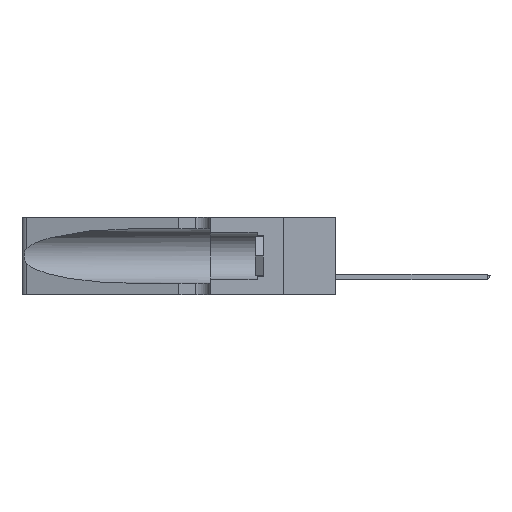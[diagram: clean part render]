
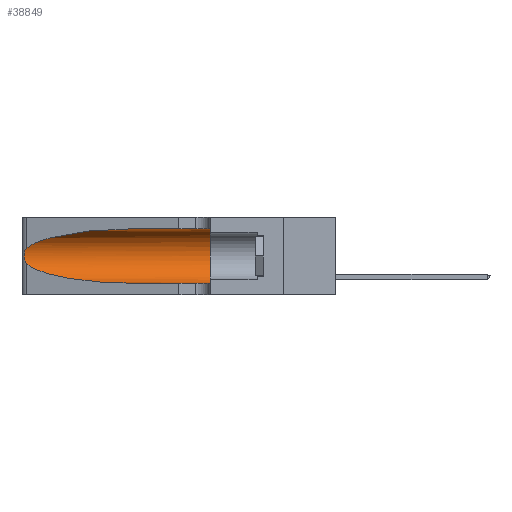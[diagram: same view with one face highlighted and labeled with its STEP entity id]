
A CAD part, left-side view. The second image highlights one B-rep face of the part: STEP entity #38849.
In plain terms, the highlighted cylindrical face has radius 3.308 mm (diameter 6.617 mm), a partial arc.
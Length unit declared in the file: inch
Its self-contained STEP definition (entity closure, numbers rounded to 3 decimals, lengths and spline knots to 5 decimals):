
#271 = DIRECTION ( 'NONE',  ( 0., 0., 1. ) ) ;
#306 = CARTESIAN_POINT ( 'NONE',  ( 0.1305, 0.72297, 0.05475 ) ) ;
#1023 = ORIENTED_EDGE ( 'NONE', *, *, #15821, .T. ) ;
#2103 =( BOUNDED_CURVE ( )  B_SPLINE_CURVE ( 3, ( #7111, #40244, #3651, #47270 ),
 .UNSPECIFIED., .F., .F. ) 
 B_SPLINE_CURVE_WITH_KNOTS ( ( 4, 4 ),
 ( 1.5708, 2.84003 ),
 .UNSPECIFIED. ) 
 CURVE ( )  GEOMETRIC_REPRESENTATION_ITEM ( )  RATIONAL_B_SPLINE_CURVE ( ( 1., 0.87, 0.87, 1. ) ) 
 REPRESENTATION_ITEM ( '' )  );
#2857 = CARTESIAN_POINT ( 'NONE',  ( 0.25487, 1.22718, 0.22369 ) ) ;
#3523 = CARTESIAN_POINT ( 'NONE',  ( 0.2373, 1.15595, 0.08982 ) ) ;
#3651 = CARTESIAN_POINT ( 'NONE',  ( 0.2373, 1.15595, 0.28018 ) ) ;
#4502 = ORIENTED_EDGE ( 'NONE', *, *, #24927, .T. ) ;
#5030 = B_SPLINE_CURVE_WITH_KNOTS ( 'NONE', 3,
 ( #2857, #31907, #13513, #46481, #17056, #17501, #28381, #6329, #13675, #28071, #20868, #9693, #6485, #28227 ),
 .UNSPECIFIED., .F., .F.,
 ( 4, 2, 2, 2, 2, 2, 4 ),
 ( 0., 0.00027, 0.00053, 0.00107, 0.0016, 0.00187, 0.00214 ),
 .UNSPECIFIED. ) ;
#6329 = CARTESIAN_POINT ( 'NONE',  ( 0.26075, 1.23896, 0.178 ) ) ;
#6485 = CARTESIAN_POINT ( 'NONE',  ( 0.25555, 1.22993, 0.14849 ) ) ;
#6826 = VERTEX_POINT ( 'NONE', #16613 ) ;
#7041 = ORIENTED_EDGE ( 'NONE', *, *, #30138, .T. ) ;
#7111 = CARTESIAN_POINT ( 'NONE',  ( 0.1305, 0.72297, 0.31525 ) ) ;
#7583 = DIRECTION ( 'NONE',  ( 0., 1., 0. ) ) ;
#8178 = VERTEX_POINT ( 'NONE', #11361 ) ;
#9440 = ORIENTED_EDGE ( 'NONE', *, *, #38004, .F. ) ;
#9693 = CARTESIAN_POINT ( 'NONE',  ( 0.25639, 1.23186, 0.15144 ) ) ;
#10323 = DIRECTION ( 'NONE',  ( 0., -1., 0. ) ) ;
#11036 = VERTEX_POINT ( 'NONE', #26827 ) ;
#11221 = CARTESIAN_POINT ( 'NONE',  ( 0.1305, 0.35, 0.31525 ) ) ;
#11361 = CARTESIAN_POINT ( 'NONE',  ( 0.1305, 0.72297, 0.31525 ) ) ;
#13513 = CARTESIAN_POINT ( 'NONE',  ( 0.25639, 1.23184, 0.21858 ) ) ;
#13675 = CARTESIAN_POINT ( 'NONE',  ( 0.26017, 1.23833, 0.17102 ) ) ;
#14470 = CIRCLE ( 'NONE', #38036, 0.13025 ) ;
#15568 = CARTESIAN_POINT ( 'NONE',  ( 0.1305, 0.72297, 0.05475 ) ) ;
#15821 = EDGE_CURVE ( 'NONE', #6826, #18283, #27553, .T. ) ;
#16191 = VERTEX_POINT ( 'NONE', #21915 ) ;
#16613 = CARTESIAN_POINT ( 'NONE',  ( 0.25487, 1.22718, 0.14631 ) ) ;
#17056 = CARTESIAN_POINT ( 'NONE',  ( 0.25854, 1.2359, 0.20912 ) ) ;
#17183 = VERTEX_POINT ( 'NONE', #11221 ) ;
#17501 = CARTESIAN_POINT ( 'NONE',  ( 0.26018, 1.23835, 0.19895 ) ) ;
#17523 = CARTESIAN_POINT ( 'NONE',  ( 0.1305, 1.61858, 0.05475 ) ) ;
#17598 = DIRECTION ( 'NONE',  ( 0., 0., -1. ) ) ;
#18283 = VERTEX_POINT ( 'NONE', #15568 ) ;
#19843 = ORIENTED_EDGE ( 'NONE', *, *, #40778, .T. ) ;
#20868 = CARTESIAN_POINT ( 'NONE',  ( 0.25789, 1.23486, 0.15765 ) ) ;
#21536 = CARTESIAN_POINT ( 'NONE',  ( 0.18966, 0.96281, 0.05475 ) ) ;
#21915 = CARTESIAN_POINT ( 'NONE',  ( 0.25487, 1.22718, 0.22369 ) ) ;
#24510 = CARTESIAN_POINT ( 'NONE',  ( 0.1305, 1.61858, 0.31525 ) ) ;
#24927 = EDGE_CURVE ( 'NONE', #16191, #6826, #5030, .T. ) ;
#25328 = LINE ( 'NONE', #24510, #40905 ) ;
#26827 = CARTESIAN_POINT ( 'NONE',  ( 0.1305, 0.35, 0.05475 ) ) ;
#27486 = LINE ( 'NONE', #17523, #35517 ) ;
#27553 =( BOUNDED_CURVE ( )  B_SPLINE_CURVE ( 3, ( #39953, #3523, #21536, #306 ),
 .UNSPECIFIED., .F., .F. ) 
 B_SPLINE_CURVE_WITH_KNOTS ( ( 4, 4 ),
 ( 3.44316, 4.71239 ),
 .UNSPECIFIED. ) 
 CURVE ( )  GEOMETRIC_REPRESENTATION_ITEM ( )  RATIONAL_B_SPLINE_CURVE ( ( 1., 0.87, 0.87, 1. ) ) 
 REPRESENTATION_ITEM ( '' )  );
#28071 = CARTESIAN_POINT ( 'NONE',  ( 0.25856, 1.23593, 0.16098 ) ) ;
#28227 = CARTESIAN_POINT ( 'NONE',  ( 0.25487, 1.22718, 0.14631 ) ) ;
#28381 = CARTESIAN_POINT ( 'NONE',  ( 0.26075, 1.23896, 0.19203 ) ) ;
#28798 = FACE_OUTER_BOUND ( 'NONE', #43531, .T. ) ;
#29632 = CARTESIAN_POINT ( 'NONE',  ( 0.1305, 0.35, 0.185 ) ) ;
#30138 = EDGE_CURVE ( 'NONE', #8178, #16191, #2103, .T. ) ;
#30474 = CYLINDRICAL_SURFACE ( 'NONE', #35574, 0.13025 ) ;
#31896 = DIRECTION ( 'NONE',  ( 0., -1., 0. ) ) ;
#31907 = CARTESIAN_POINT ( 'NONE',  ( 0.25555, 1.22994, 0.2215 ) ) ;
#35517 = VECTOR ( 'NONE', #10323, 39.37008 ) ;
#35574 = AXIS2_PLACEMENT_3D ( 'NONE', #40023, #47379, #17598 ) ;
#38004 = EDGE_CURVE ( 'NONE', #8178, #17183, #25328, .T. ) ;
#38036 = AXIS2_PLACEMENT_3D ( 'NONE', #29632, #7583, #271 ) ;
#38239 = EDGE_CURVE ( 'NONE', #17183, #11036, #14470, .T. ) ;
#38458 = ORIENTED_EDGE ( 'NONE', *, *, #38239, .F. ) ;
#38849 = ADVANCED_FACE ( 'NONE', ( #28798 ), #30474, .F. ) ;
#39953 = CARTESIAN_POINT ( 'NONE',  ( 0.25487, 1.22718, 0.14631 ) ) ;
#40023 = CARTESIAN_POINT ( 'NONE',  ( 0.1305, 1.61858, 0.185 ) ) ;
#40244 = CARTESIAN_POINT ( 'NONE',  ( 0.18966, 0.96281, 0.31525 ) ) ;
#40778 = EDGE_CURVE ( 'NONE', #18283, #11036, #27486, .T. ) ;
#40905 = VECTOR ( 'NONE', #31896, 39.37008 ) ;
#43531 = EDGE_LOOP ( 'NONE', ( #7041, #4502, #1023, #19843, #38458, #9440 ) ) ;
#46481 = CARTESIAN_POINT ( 'NONE',  ( 0.25787, 1.23484, 0.2124 ) ) ;
#47270 = CARTESIAN_POINT ( 'NONE',  ( 0.25487, 1.22718, 0.22369 ) ) ;
#47379 = DIRECTION ( 'NONE',  ( 0., -1., 0. ) ) ;
